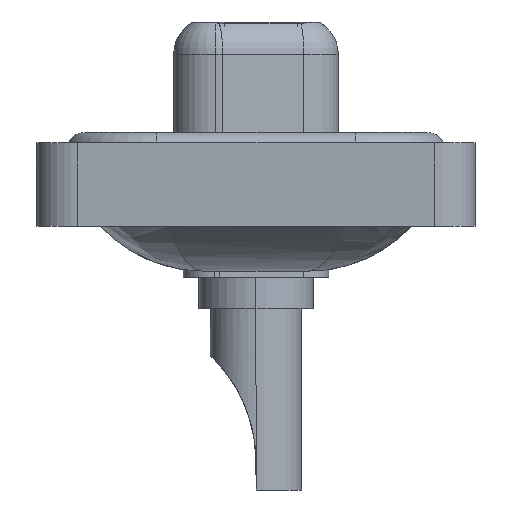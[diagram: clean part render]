
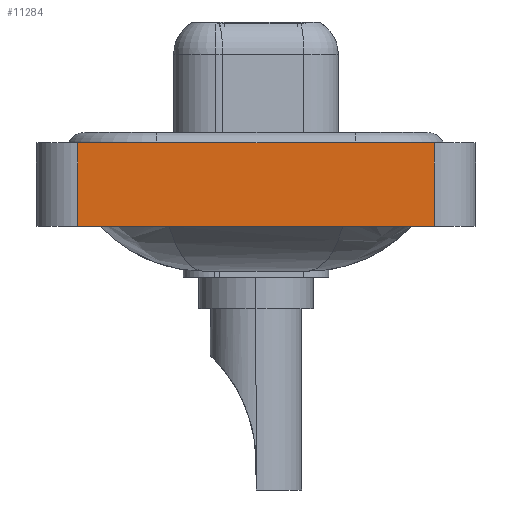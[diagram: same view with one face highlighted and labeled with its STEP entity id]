
A CAD part, left-side view. The second image highlights one B-rep face of the part: STEP entity #11284.
In plain terms, the highlighted planar face has unit normal (-1, 0, 0).
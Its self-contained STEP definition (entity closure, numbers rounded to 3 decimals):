
#277 = LINE ( 'NONE', #10001, #3197 ) ;
#2468 = DIRECTION ( 'NONE',  ( 0., 0., 1. ) ) ;
#3197 = VECTOR ( 'NONE', #21105, 1000. ) ;
#5664 = VECTOR ( 'NONE', #17054, 1000. ) ;
#5685 = LINE ( 'NONE', #23237, #5664 ) ;
#6372 = DIRECTION ( 'NONE',  ( -1., 0., 0. ) ) ;
#6512 = LINE ( 'NONE', #21941, #14349 ) ;
#7536 = LINE ( 'NONE', #19282, #18461 ) ;
#7752 = ORIENTED_EDGE ( 'NONE', *, *, #19405, .T. ) ;
#9284 = EDGE_LOOP ( 'NONE', ( #19067, #11904, #23599, #7752 ) ) ;
#9472 = EDGE_CURVE ( 'NONE', #12549, #20749, #6512, .T. ) ;
#10001 = CARTESIAN_POINT ( 'NONE',  ( -7.35, -8.55, -3.6 ) ) ;
#10178 = PLANE ( 'NONE',  #13621 ) ;
#11052 = EDGE_CURVE ( 'NONE', #15493, #12549, #7536, .T. ) ;
#11284 = ADVANCED_FACE ( 'NONE', ( #21673 ), #10178, .T. ) ;
#11904 = ORIENTED_EDGE ( 'NONE', *, *, #9472, .F. ) ;
#12325 = CARTESIAN_POINT ( 'NONE',  ( -7.35, -8.55, -3.6 ) ) ;
#12349 = DIRECTION ( 'NONE',  ( 0., -1., 0. ) ) ;
#12549 = VERTEX_POINT ( 'NONE', #17987 ) ;
#13229 = DIRECTION ( 'NONE',  ( 0., 0., 1. ) ) ;
#13621 = AXIS2_PLACEMENT_3D ( 'NONE', #12325, #6372, #2468 ) ;
#14349 = VECTOR ( 'NONE', #12349, 1000. ) ;
#15493 = VERTEX_POINT ( 'NONE', #17644 ) ;
#17054 = DIRECTION ( 'NONE',  ( 0., -1., 0. ) ) ;
#17644 = CARTESIAN_POINT ( 'NONE',  ( -7.35, 8.55, -3.6 ) ) ;
#17926 = EDGE_CURVE ( 'NONE', #19271, #20749, #277, .T. ) ;
#17987 = CARTESIAN_POINT ( 'NONE',  ( -7.35, 8.55, 0.4 ) ) ;
#18461 = VECTOR ( 'NONE', #13229, 1000. ) ;
#19067 = ORIENTED_EDGE ( 'NONE', *, *, #17926, .T. ) ;
#19271 = VERTEX_POINT ( 'NONE', #20225 ) ;
#19282 = CARTESIAN_POINT ( 'NONE',  ( -7.35, 8.55, -3.6 ) ) ;
#19355 = CARTESIAN_POINT ( 'NONE',  ( -7.35, -8.55, 0.4 ) ) ;
#19405 = EDGE_CURVE ( 'NONE', #15493, #19271, #5685, .T. ) ;
#20225 = CARTESIAN_POINT ( 'NONE',  ( -7.35, -8.55, -3.6 ) ) ;
#20749 = VERTEX_POINT ( 'NONE', #19355 ) ;
#21105 = DIRECTION ( 'NONE',  ( 0., 0., 1. ) ) ;
#21673 = FACE_OUTER_BOUND ( 'NONE', #9284, .T. ) ;
#21941 = CARTESIAN_POINT ( 'NONE',  ( -7.35, -8.55, 0.4 ) ) ;
#23237 = CARTESIAN_POINT ( 'NONE',  ( -7.35, -8.55, -3.6 ) ) ;
#23599 = ORIENTED_EDGE ( 'NONE', *, *, #11052, .F. ) ;
